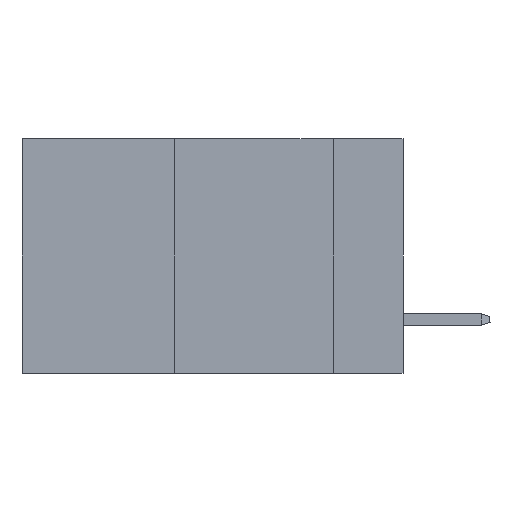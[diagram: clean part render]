
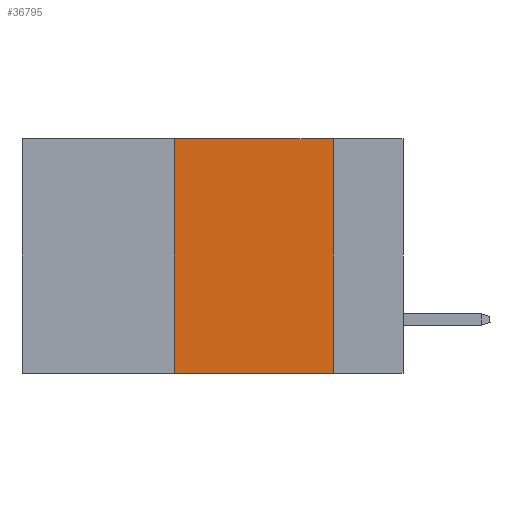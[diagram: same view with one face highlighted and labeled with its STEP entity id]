
A CAD part, left-side view. The second image highlights one B-rep face of the part: STEP entity #36795.
In plain terms, the highlighted planar face has unit normal (-1, 0, 0).
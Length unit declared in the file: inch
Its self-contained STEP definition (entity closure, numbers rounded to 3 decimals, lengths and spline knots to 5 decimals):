
#371 = LINE ( 'NONE', #26128, #5279 ) ;
#2656 = ORIENTED_EDGE ( 'NONE', *, *, #11215, .F. ) ;
#2785 = DIRECTION ( 'NONE',  ( 1., 0., 0. ) ) ;
#3502 = VECTOR ( 'NONE', #19191, 39.37008 ) ;
#4507 = EDGE_CURVE ( 'NONE', #29837, #27688, #371, .T. ) ;
#5279 = VECTOR ( 'NONE', #22111, 39.37008 ) ;
#6785 = VERTEX_POINT ( 'NONE', #19392 ) ;
#7017 = CARTESIAN_POINT ( 'NONE',  ( 0., 0.11, -0.37 ) ) ;
#7233 = LINE ( 'NONE', #43344, #34552 ) ;
#11215 = EDGE_CURVE ( 'NONE', #6785, #38075, #18378, .T. ) ;
#14598 = VECTOR ( 'NONE', #21696, 39.37008 ) ;
#15542 = CARTESIAN_POINT ( 'NONE',  ( 0., 0.36, 0. ) ) ;
#18327 = DIRECTION ( 'NONE',  ( 0., -1., 0. ) ) ;
#18378 = LINE ( 'NONE', #39629, #14598 ) ;
#19191 = DIRECTION ( 'NONE',  ( 0., -1., 0. ) ) ;
#19198 = ORIENTED_EDGE ( 'NONE', *, *, #32275, .F. ) ;
#19392 = CARTESIAN_POINT ( 'NONE',  ( 0., 0.11, 0. ) ) ;
#19638 = ORIENTED_EDGE ( 'NONE', *, *, #30608, .T. ) ;
#20485 = FACE_OUTER_BOUND ( 'NONE', #20564, .T. ) ;
#20564 = EDGE_LOOP ( 'NONE', ( #2656, #19198, #28532, #19638 ) ) ;
#21418 = DIRECTION ( 'NONE',  ( 0., 0., -1. ) ) ;
#21696 = DIRECTION ( 'NONE',  ( 0., 0., -1. ) ) ;
#22111 = DIRECTION ( 'NONE',  ( 0., 0., 1. ) ) ;
#26128 = CARTESIAN_POINT ( 'NONE',  ( 0., 0.36, 0. ) ) ;
#27688 = VERTEX_POINT ( 'NONE', #15542 ) ;
#28509 = PLANE ( 'NONE',  #32461 ) ;
#28532 = ORIENTED_EDGE ( 'NONE', *, *, #4507, .F. ) ;
#29837 = VERTEX_POINT ( 'NONE', #34908 ) ;
#30608 = EDGE_CURVE ( 'NONE', #29837, #38075, #44190, .T. ) ;
#31358 = CARTESIAN_POINT ( 'NONE',  ( 0., 0.6, 0. ) ) ;
#32275 = EDGE_CURVE ( 'NONE', #27688, #6785, #7233, .T. ) ;
#32461 = AXIS2_PLACEMENT_3D ( 'NONE', #31358, #2785, #21418 ) ;
#34552 = VECTOR ( 'NONE', #18327, 39.37008 ) ;
#34908 = CARTESIAN_POINT ( 'NONE',  ( 0., 0.36, -0.37 ) ) ;
#36795 = ADVANCED_FACE ( 'NONE', ( #20485 ), #28509, .F. ) ;
#38075 = VERTEX_POINT ( 'NONE', #7017 ) ;
#39629 = CARTESIAN_POINT ( 'NONE',  ( 0., 0.11, 0. ) ) ;
#43344 = CARTESIAN_POINT ( 'NONE',  ( 0., 0.6, 0. ) ) ;
#44190 = LINE ( 'NONE', #44658, #3502 ) ;
#44658 = CARTESIAN_POINT ( 'NONE',  ( 0., 0.6, -0.37 ) ) ;
